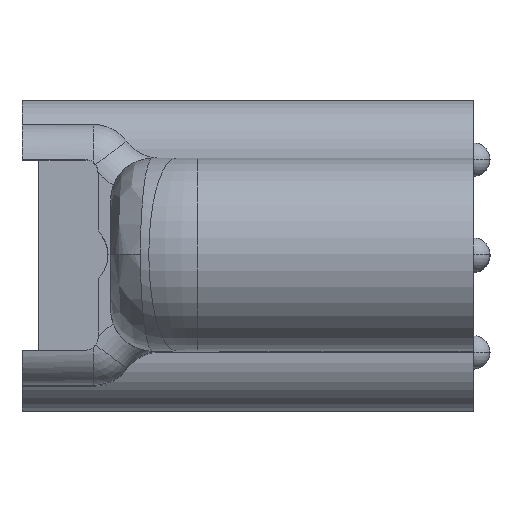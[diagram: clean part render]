
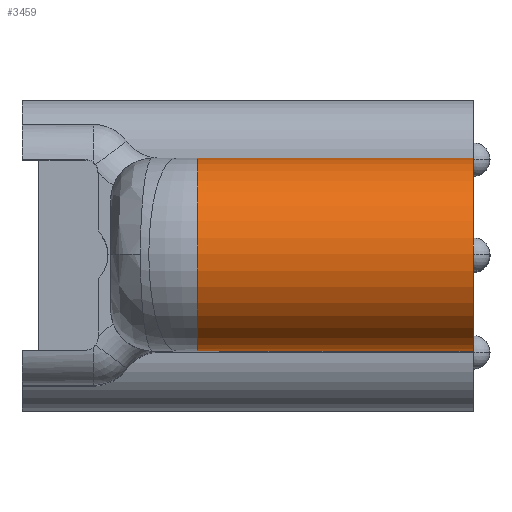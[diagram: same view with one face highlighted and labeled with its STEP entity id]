
A CAD part, top view. The second image highlights one B-rep face of the part: STEP entity #3459.
In plain terms, the highlighted cylindrical face has radius 11.509 mm (diameter 23.019 mm), a partial arc.
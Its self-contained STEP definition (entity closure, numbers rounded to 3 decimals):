
#433 = AXIS2_PLACEMENT_3D ( 'NONE', #3712, #3717, #3736 ) ;
#584 = EDGE_CURVE ( 'NONE', #3813, #2812, #1009, .T. ) ;
#593 = EDGE_CURVE ( 'NONE', #3868, #2812, #1018, .T. ) ;
#635 = CARTESIAN_POINT ( 'NONE',  ( -38.699, -61.776, 47.014 ) ) ;
#655 = EDGE_CURVE ( 'NONE', #3813, #1235, #903, .T. ) ;
#716 = DIRECTION ( 'NONE',  ( 0., -1., 0. ) ) ;
#804 = DIRECTION ( 'NONE',  ( 1., 0., 0. ) ) ;
#892 = VECTOR ( 'NONE', #2269, 1000. ) ;
#903 = LINE ( 'NONE', #2264, #892 ) ;
#955 = DIRECTION ( 'NONE',  ( 0., 0., -1. ) ) ;
#974 = DIRECTION ( 'NONE',  ( -1., 0., 0. ) ) ;
#988 = CARTESIAN_POINT ( 'NONE',  ( -42.818, -61.776, 47.014 ) ) ;
#994 = VECTOR ( 'NONE', #2656, 1000. ) ;
#1009 = CIRCLE ( 'NONE', #433, 11.509 ) ;
#1018 = LINE ( 'NONE', #3751, #994 ) ;
#1063 = CARTESIAN_POINT ( 'NONE',  ( -42.818, -50.267, 47.014 ) ) ;
#1235 = VERTEX_POINT ( 'NONE', #1063 ) ;
#1608 = EDGE_CURVE ( 'NONE', #3868, #1235, #2515, .T. ) ;
#2118 = EDGE_LOOP ( 'NONE', ( #3466, #3359, #3283, #3576 ) ) ;
#2264 = CARTESIAN_POINT ( 'NONE',  ( -38.699, -50.267, 47.014 ) ) ;
#2269 = DIRECTION ( 'NONE',  ( 1., 0., 0. ) ) ;
#2374 = CARTESIAN_POINT ( 'NONE',  ( -75.74, -73.285, 47.014 ) ) ;
#2515 = CIRCLE ( 'NONE', #3266, 11.509 ) ;
#2656 = DIRECTION ( 'NONE',  ( -1., 0., 0. ) ) ;
#2812 = VERTEX_POINT ( 'NONE', #2374 ) ;
#2874 = CARTESIAN_POINT ( 'NONE',  ( -42.818, -73.285, 47.014 ) ) ;
#2953 = CARTESIAN_POINT ( 'NONE',  ( -75.74, -50.267, 47.014 ) ) ;
#3127 = CYLINDRICAL_SURFACE ( 'NONE', #3272, 11.509 ) ;
#3266 = AXIS2_PLACEMENT_3D ( 'NONE', #988, #974, #955 ) ;
#3272 = AXIS2_PLACEMENT_3D ( 'NONE', #635, #804, #716 ) ;
#3283 = ORIENTED_EDGE ( 'NONE', *, *, #655, .F. ) ;
#3359 = ORIENTED_EDGE ( 'NONE', *, *, #1608, .T. ) ;
#3459 = ADVANCED_FACE ( 'NONE', ( #3897 ), #3127, .T. ) ;
#3466 = ORIENTED_EDGE ( 'NONE', *, *, #593, .F. ) ;
#3576 = ORIENTED_EDGE ( 'NONE', *, *, #584, .T. ) ;
#3712 = CARTESIAN_POINT ( 'NONE',  ( -75.74, -61.776, 47.014 ) ) ;
#3717 = DIRECTION ( 'NONE',  ( 1., 0., 0. ) ) ;
#3736 = DIRECTION ( 'NONE',  ( 0., -1., 0. ) ) ;
#3751 = CARTESIAN_POINT ( 'NONE',  ( 59.385, -73.285, 47.014 ) ) ;
#3813 = VERTEX_POINT ( 'NONE', #2953 ) ;
#3868 = VERTEX_POINT ( 'NONE', #2874 ) ;
#3897 = FACE_OUTER_BOUND ( 'NONE', #2118, .T. ) ;
